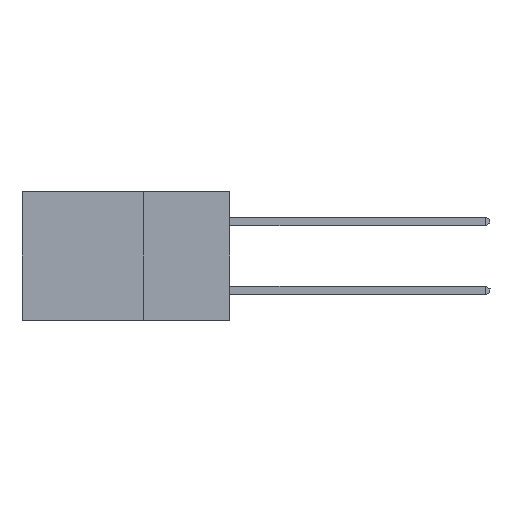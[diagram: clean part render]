
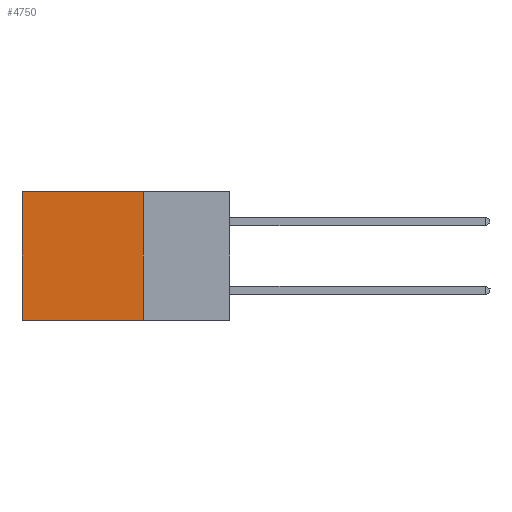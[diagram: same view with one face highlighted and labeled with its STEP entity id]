
A CAD part, left-side view. The second image highlights one B-rep face of the part: STEP entity #4750.
In plain terms, the highlighted planar face has unit normal (-1, 0, 0).
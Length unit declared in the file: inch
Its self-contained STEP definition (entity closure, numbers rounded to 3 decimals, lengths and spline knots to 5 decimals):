
#742 = EDGE_CURVE ( 'NONE', #14615, #3267, #13311, .T. ) ;
#806 = DIRECTION ( 'NONE',  ( 0., 0., -1. ) ) ;
#1376 = LINE ( 'NONE', #23793, #16708 ) ;
#1924 = DIRECTION ( 'NONE',  ( 0., 0., -1. ) ) ;
#3267 = VERTEX_POINT ( 'NONE', #13552 ) ;
#4393 = VECTOR ( 'NONE', #9797, 39.37008 ) ;
#4750 = ADVANCED_FACE ( 'NONE', ( #21543 ), #5921, .F. ) ;
#5767 = VECTOR ( 'NONE', #23114, 39.37008 ) ;
#5921 = PLANE ( 'NONE',  #7043 ) ;
#6568 = CARTESIAN_POINT ( 'NONE',  ( 0.298, 0.25, 0. ) ) ;
#7043 = AXIS2_PLACEMENT_3D ( 'NONE', #19875, #19627, #7899 ) ;
#7899 = DIRECTION ( 'NONE',  ( 0., 0., -1. ) ) ;
#9510 = CARTESIAN_POINT ( 'NONE',  ( 0.298, 0.25, -0.37 ) ) ;
#9719 = CARTESIAN_POINT ( 'NONE',  ( 0.298, 0.25, 0. ) ) ;
#9797 = DIRECTION ( 'NONE',  ( 0., 1., 0. ) ) ;
#9838 = VECTOR ( 'NONE', #806, 39.37008 ) ;
#11368 = EDGE_CURVE ( 'NONE', #3267, #21518, #1376, .T. ) ;
#13261 = EDGE_CURVE ( 'NONE', #14615, #16360, #21462, .T. ) ;
#13311 = LINE ( 'NONE', #9719, #4393 ) ;
#13552 = CARTESIAN_POINT ( 'NONE',  ( 0.298, 0.6, 0. ) ) ;
#14615 = VERTEX_POINT ( 'NONE', #6568 ) ;
#15064 = CARTESIAN_POINT ( 'NONE',  ( 0.298, 0.6, -0.37 ) ) ;
#16360 = VERTEX_POINT ( 'NONE', #18788 ) ;
#16612 = CARTESIAN_POINT ( 'NONE',  ( 0.298, 0.25, 0. ) ) ;
#16708 = VECTOR ( 'NONE', #1924, 39.37008 ) ;
#16868 = ORIENTED_EDGE ( 'NONE', *, *, #13261, .F. ) ;
#17529 = EDGE_CURVE ( 'NONE', #16360, #21518, #23538, .T. ) ;
#18788 = CARTESIAN_POINT ( 'NONE',  ( 0.298, 0.25, -0.37 ) ) ;
#19037 = ORIENTED_EDGE ( 'NONE', *, *, #17529, .F. ) ;
#19627 = DIRECTION ( 'NONE',  ( 1., 0., 0. ) ) ;
#19875 = CARTESIAN_POINT ( 'NONE',  ( 0.298, 0.25, 0. ) ) ;
#21462 = LINE ( 'NONE', #16612, #9838 ) ;
#21518 = VERTEX_POINT ( 'NONE', #15064 ) ;
#21543 = FACE_OUTER_BOUND ( 'NONE', #25096, .T. ) ;
#23114 = DIRECTION ( 'NONE',  ( 0., 1., 0. ) ) ;
#23538 = LINE ( 'NONE', #9510, #5767 ) ;
#23588 = ORIENTED_EDGE ( 'NONE', *, *, #742, .T. ) ;
#23793 = CARTESIAN_POINT ( 'NONE',  ( 0.298, 0.6, 0. ) ) ;
#24714 = ORIENTED_EDGE ( 'NONE', *, *, #11368, .T. ) ;
#25096 = EDGE_LOOP ( 'NONE', ( #24714, #19037, #16868, #23588 ) ) ;
